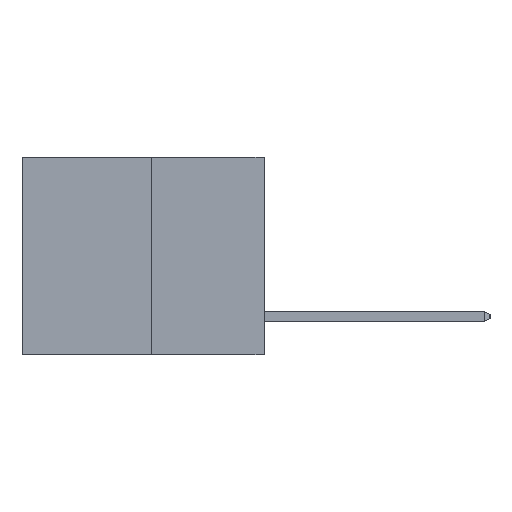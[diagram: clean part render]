
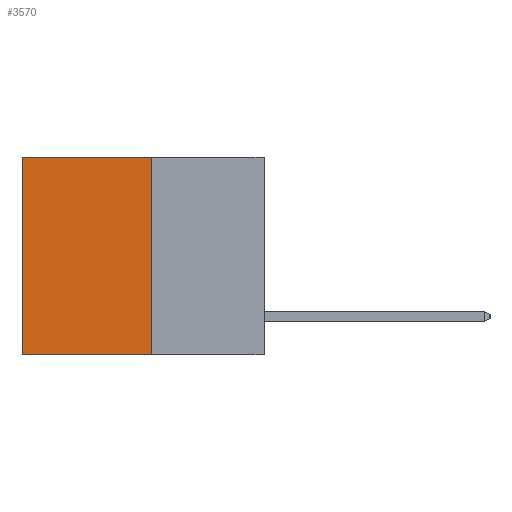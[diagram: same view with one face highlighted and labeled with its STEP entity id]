
A CAD part, left-side view. The second image highlights one B-rep face of the part: STEP entity #3570.
In plain terms, the highlighted planar face has unit normal (-1, 0, 0).
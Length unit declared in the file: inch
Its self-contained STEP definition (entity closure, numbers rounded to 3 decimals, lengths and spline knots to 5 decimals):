
#28 = CARTESIAN_POINT ( 'NONE',  ( 0.3165, 0.6, -0.49 ) ) ;
#132 = DIRECTION ( 'NONE',  ( 0., 0., -1. ) ) ;
#189 = VECTOR ( 'NONE', #1736, 39.37008 ) ;
#1057 = ORIENTED_EDGE ( 'NONE', *, *, #9566, .T. ) ;
#1156 = VECTOR ( 'NONE', #132, 39.37008 ) ;
#1736 = DIRECTION ( 'NONE',  ( 0., 1., 0. ) ) ;
#1825 = EDGE_LOOP ( 'NONE', ( #8061, #1843, #8926, #1057 ) ) ;
#1843 = ORIENTED_EDGE ( 'NONE', *, *, #5025, .F. ) ;
#1849 = LINE ( 'NONE', #2525, #189 ) ;
#2447 = DIRECTION ( 'NONE',  ( 0., 0., -1. ) ) ;
#2462 = LINE ( 'NONE', #6470, #8874 ) ;
#2525 = CARTESIAN_POINT ( 'NONE',  ( 0.3165, 0.28, -0.49 ) ) ;
#3145 = PLANE ( 'NONE',  #3656 ) ;
#3389 = VERTEX_POINT ( 'NONE', #10576 ) ;
#3570 = ADVANCED_FACE ( 'NONE', ( #9462 ), #3145, .F. ) ;
#3656 = AXIS2_PLACEMENT_3D ( 'NONE', #8191, #7464, #2447 ) ;
#4561 = CARTESIAN_POINT ( 'NONE',  ( 0.3165, 0.28, -0.49 ) ) ;
#5025 = EDGE_CURVE ( 'NONE', #9761, #3389, #1849, .T. ) ;
#6067 = LINE ( 'NONE', #6145, #7256 ) ;
#6145 = CARTESIAN_POINT ( 'NONE',  ( 0.3165, 0.28, 0. ) ) ;
#6423 = VERTEX_POINT ( 'NONE', #9890 ) ;
#6470 = CARTESIAN_POINT ( 'NONE',  ( 0.3165, 0.28, -0.49 ) ) ;
#6650 = CARTESIAN_POINT ( 'NONE',  ( 0.3165, 0.28, 0. ) ) ;
#6954 = VERTEX_POINT ( 'NONE', #6650 ) ;
#6990 = DIRECTION ( 'NONE',  ( 0., 1., 0. ) ) ;
#7256 = VECTOR ( 'NONE', #6990, 39.37008 ) ;
#7464 = DIRECTION ( 'NONE',  ( 1., 0., 0. ) ) ;
#8061 = ORIENTED_EDGE ( 'NONE', *, *, #9426, .T. ) ;
#8131 = DIRECTION ( 'NONE',  ( 0., 0., -1. ) ) ;
#8191 = CARTESIAN_POINT ( 'NONE',  ( 0.3165, 0.28, -0.49 ) ) ;
#8441 = LINE ( 'NONE', #28, #1156 ) ;
#8874 = VECTOR ( 'NONE', #8131, 39.37008 ) ;
#8926 = ORIENTED_EDGE ( 'NONE', *, *, #9190, .F. ) ;
#9190 = EDGE_CURVE ( 'NONE', #6954, #9761, #2462, .T. ) ;
#9426 = EDGE_CURVE ( 'NONE', #6423, #3389, #8441, .T. ) ;
#9462 = FACE_OUTER_BOUND ( 'NONE', #1825, .T. ) ;
#9566 = EDGE_CURVE ( 'NONE', #6954, #6423, #6067, .T. ) ;
#9761 = VERTEX_POINT ( 'NONE', #4561 ) ;
#9890 = CARTESIAN_POINT ( 'NONE',  ( 0.3165, 0.6, 0. ) ) ;
#10576 = CARTESIAN_POINT ( 'NONE',  ( 0.3165, 0.6, -0.49 ) ) ;
